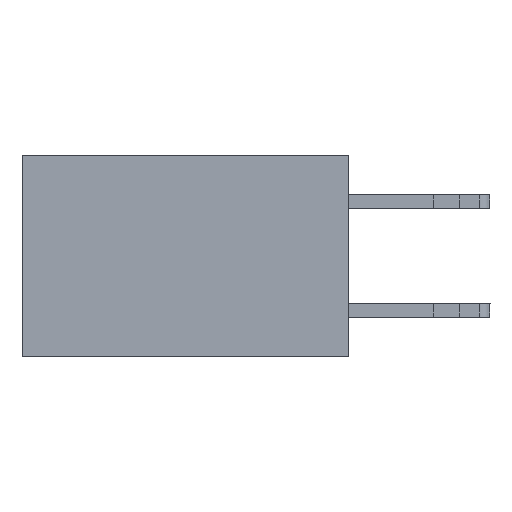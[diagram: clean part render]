
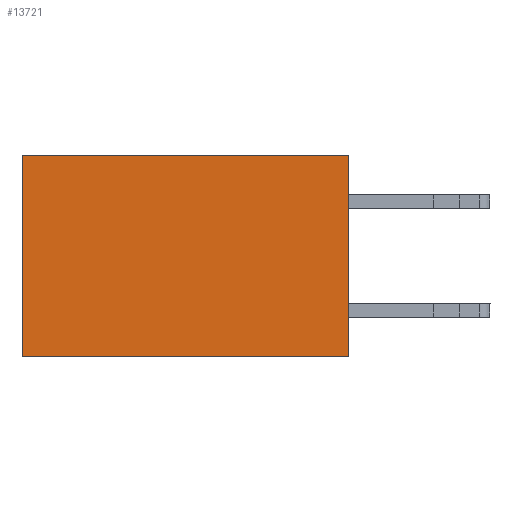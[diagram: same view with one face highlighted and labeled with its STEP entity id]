
A CAD part, left-side view. The second image highlights one B-rep face of the part: STEP entity #13721.
In plain terms, the highlighted planar face has unit normal (-1, 0, 0).
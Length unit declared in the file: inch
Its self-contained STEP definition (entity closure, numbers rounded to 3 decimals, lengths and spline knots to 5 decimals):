
#729 = ORIENTED_EDGE ( 'NONE', *, *, #12712, .T. ) ;
#976 = VERTEX_POINT ( 'NONE', #8928 ) ;
#1025 = VECTOR ( 'NONE', #12443, 39.37008 ) ;
#1202 = EDGE_LOOP ( 'NONE', ( #7342, #13737, #8533, #729 ) ) ;
#1424 = VERTEX_POINT ( 'NONE', #13308 ) ;
#2685 = PLANE ( 'NONE',  #2699 ) ;
#2699 = AXIS2_PLACEMENT_3D ( 'NONE', #6186, #14188, #7287 ) ;
#2750 = VERTEX_POINT ( 'NONE', #13672 ) ;
#2762 = LINE ( 'NONE', #5261, #8449 ) ;
#3314 = EDGE_CURVE ( 'NONE', #976, #1424, #8834, .T. ) ;
#3823 = EDGE_CURVE ( 'NONE', #1424, #7421, #2762, .T. ) ;
#4155 = LINE ( 'NONE', #5589, #1025 ) ;
#5241 = DIRECTION ( 'NONE',  ( 0., 1., 0. ) ) ;
#5261 = CARTESIAN_POINT ( 'NONE',  ( 0.2615, 0., -0.37 ) ) ;
#5589 = CARTESIAN_POINT ( 'NONE',  ( 0.2615, 0., 0. ) ) ;
#5876 = VECTOR ( 'NONE', #9305, 39.37008 ) ;
#6186 = CARTESIAN_POINT ( 'NONE',  ( 0.2615, 0., -0.37 ) ) ;
#7287 = DIRECTION ( 'NONE',  ( 0., 0., -1. ) ) ;
#7342 = ORIENTED_EDGE ( 'NONE', *, *, #10192, .T. ) ;
#7421 = VERTEX_POINT ( 'NONE', #12900 ) ;
#7497 = VECTOR ( 'NONE', #10311, 39.37008 ) ;
#7984 = FACE_OUTER_BOUND ( 'NONE', #1202, .T. ) ;
#8449 = VECTOR ( 'NONE', #5241, 39.37008 ) ;
#8533 = ORIENTED_EDGE ( 'NONE', *, *, #3314, .F. ) ;
#8834 = LINE ( 'NONE', #9114, #5876 ) ;
#8928 = CARTESIAN_POINT ( 'NONE',  ( 0.2615, 0., 0. ) ) ;
#9078 = CARTESIAN_POINT ( 'NONE',  ( 0.2615, 0.6, -0.37 ) ) ;
#9114 = CARTESIAN_POINT ( 'NONE',  ( 0.2615, 0., -0.37 ) ) ;
#9305 = DIRECTION ( 'NONE',  ( 0., 0., -1. ) ) ;
#10192 = EDGE_CURVE ( 'NONE', #2750, #7421, #10616, .T. ) ;
#10311 = DIRECTION ( 'NONE',  ( 0., 0., -1. ) ) ;
#10616 = LINE ( 'NONE', #9078, #7497 ) ;
#12443 = DIRECTION ( 'NONE',  ( 0., 1., 0. ) ) ;
#12712 = EDGE_CURVE ( 'NONE', #976, #2750, #4155, .T. ) ;
#12900 = CARTESIAN_POINT ( 'NONE',  ( 0.2615, 0.6, -0.37 ) ) ;
#13308 = CARTESIAN_POINT ( 'NONE',  ( 0.2615, 0., -0.37 ) ) ;
#13672 = CARTESIAN_POINT ( 'NONE',  ( 0.2615, 0.6, 0. ) ) ;
#13721 = ADVANCED_FACE ( 'NONE', ( #7984 ), #2685, .F. ) ;
#13737 = ORIENTED_EDGE ( 'NONE', *, *, #3823, .F. ) ;
#14188 = DIRECTION ( 'NONE',  ( 1., 0., 0. ) ) ;
